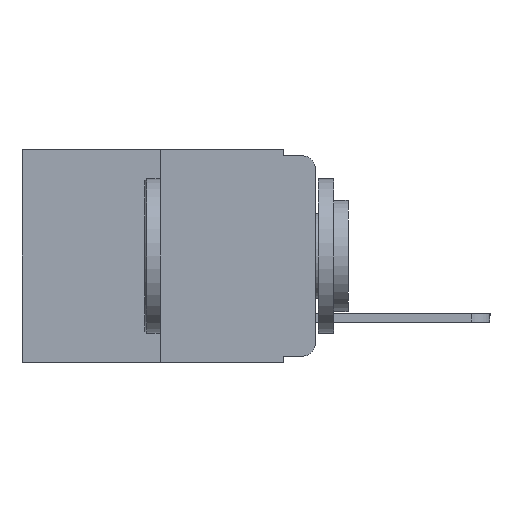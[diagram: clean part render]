
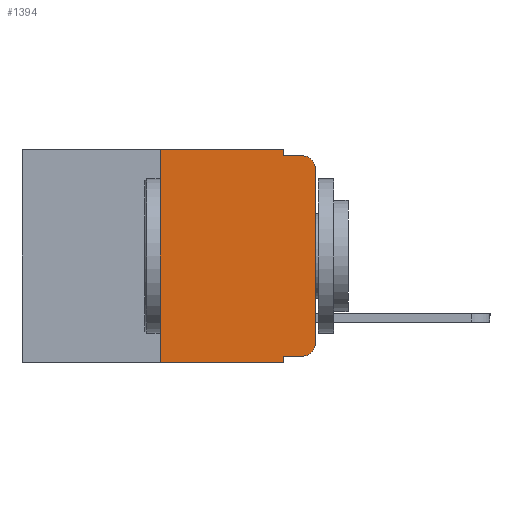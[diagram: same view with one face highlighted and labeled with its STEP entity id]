
A CAD part, left-side view. The second image highlights one B-rep face of the part: STEP entity #1394.
In plain terms, the highlighted planar face has unit normal (-1, 0, 0).
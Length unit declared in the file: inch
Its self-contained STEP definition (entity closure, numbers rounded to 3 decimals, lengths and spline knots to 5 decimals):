
#51 = CARTESIAN_POINT ( 'NONE',  ( 0., 0.051, -0.333 ) ) ;
#210 = EDGE_CURVE ( 'NONE', #1624, #1306, #15572, .T. ) ;
#361 = DIRECTION ( 'NONE',  ( 0., -1., 0. ) ) ;
#1216 = EDGE_CURVE ( 'NONE', #1306, #7808, #3694, .T. ) ;
#1306 = VERTEX_POINT ( 'NONE', #14944 ) ;
#1387 = DIRECTION ( 'NONE',  ( -1., 0., 0. ) ) ;
#1394 = ADVANCED_FACE ( 'NONE', ( #12796 ), #8373, .F. ) ;
#1551 = VERTEX_POINT ( 'NONE', #9295 ) ;
#1624 = VERTEX_POINT ( 'NONE', #13946 ) ;
#1901 = CARTESIAN_POINT ( 'NONE',  ( 0., 0., -0.03 ) ) ;
#1921 = VERTEX_POINT ( 'NONE', #14978 ) ;
#2277 = VERTEX_POINT ( 'NONE', #6408 ) ;
#2470 = CARTESIAN_POINT ( 'NONE',  ( 0., 0.25, -0.343 ) ) ;
#3202 = VERTEX_POINT ( 'NONE', #1901 ) ;
#3694 = CIRCLE ( 'NONE', #9888, 0.02 ) ;
#3838 = DIRECTION ( 'NONE',  ( 0., -1., 0. ) ) ;
#4128 = EDGE_CURVE ( 'NONE', #7808, #3202, #12061, .T. ) ;
#4379 = CARTESIAN_POINT ( 'NONE',  ( 0., 0.051, -0.343 ) ) ;
#4823 = VERTEX_POINT ( 'NONE', #4379 ) ;
#4989 = VERTEX_POINT ( 'NONE', #11772 ) ;
#5062 = LINE ( 'NONE', #13606, #20707 ) ;
#6408 = CARTESIAN_POINT ( 'NONE',  ( 0., 0.051, -0.01 ) ) ;
#6953 = DIRECTION ( 'NONE',  ( 0., -1., 0. ) ) ;
#7467 = DIRECTION ( 'NONE',  ( 0., -1., 0. ) ) ;
#7548 = EDGE_CURVE ( 'NONE', #8425, #4823, #14599, .T. ) ;
#7808 = VERTEX_POINT ( 'NONE', #11474 ) ;
#7909 = VECTOR ( 'NONE', #17127, 39.37008 ) ;
#7979 = CIRCLE ( 'NONE', #13161, 0.02 ) ;
#8373 = PLANE ( 'NONE',  #13572 ) ;
#8418 = VECTOR ( 'NONE', #6953, 39.37008 ) ;
#8425 = VERTEX_POINT ( 'NONE', #2470 ) ;
#8596 = EDGE_CURVE ( 'NONE', #2277, #1921, #5062, .T. ) ;
#8642 = CARTESIAN_POINT ( 'NONE',  ( 0., 0.473, 0. ) ) ;
#9066 = LINE ( 'NONE', #17941, #16503 ) ;
#9295 = CARTESIAN_POINT ( 'NONE',  ( 0., 0.25, 0. ) ) ;
#9774 = CARTESIAN_POINT ( 'NONE',  ( 0., 0., 0. ) ) ;
#9883 = EDGE_CURVE ( 'NONE', #1624, #4823, #9066, .T. ) ;
#9888 = AXIS2_PLACEMENT_3D ( 'NONE', #16943, #16154, #15455 ) ;
#10025 = EDGE_LOOP ( 'NONE', ( #12259, #12470, #12678, #12743, #12898, #12948, #13164, #13176, #13274, #13367 ) ) ;
#10623 = VECTOR ( 'NONE', #361, 39.37008 ) ;
#10733 = VECTOR ( 'NONE', #18582, 39.37008 ) ;
#10994 = CARTESIAN_POINT ( 'NONE',  ( 0., 0.473, -0.343 ) ) ;
#11474 = CARTESIAN_POINT ( 'NONE',  ( 0., 0., -0.313 ) ) ;
#11691 = VECTOR ( 'NONE', #3838, 39.37008 ) ;
#11772 = CARTESIAN_POINT ( 'NONE',  ( 0., 0.051, 0. ) ) ;
#11783 = CARTESIAN_POINT ( 'NONE',  ( 0., 0.02, -0.03 ) ) ;
#12061 = LINE ( 'NONE', #9774, #7909 ) ;
#12259 = ORIENTED_EDGE ( 'NONE', *, *, #4128, .T. ) ;
#12345 = VECTOR ( 'NONE', #13109, 39.37008 ) ;
#12470 = ORIENTED_EDGE ( 'NONE', *, *, #18133, .T. ) ;
#12678 = ORIENTED_EDGE ( 'NONE', *, *, #8596, .F. ) ;
#12743 = ORIENTED_EDGE ( 'NONE', *, *, #16344, .F. ) ;
#12796 = FACE_OUTER_BOUND ( 'NONE', #10025, .T. ) ;
#12810 = LINE ( 'NONE', #20193, #12345 ) ;
#12898 = ORIENTED_EDGE ( 'NONE', *, *, #19714, .F. ) ;
#12948 = ORIENTED_EDGE ( 'NONE', *, *, #17063, .F. ) ;
#13001 = LINE ( 'NONE', #8642, #8418 ) ;
#13109 = DIRECTION ( 'NONE',  ( 0., 0., -1. ) ) ;
#13132 = CARTESIAN_POINT ( 'NONE',  ( 0., 0.473, 0. ) ) ;
#13161 = AXIS2_PLACEMENT_3D ( 'NONE', #11783, #1387, #13255 ) ;
#13164 = ORIENTED_EDGE ( 'NONE', *, *, #7548, .T. ) ;
#13176 = ORIENTED_EDGE ( 'NONE', *, *, #9883, .F. ) ;
#13231 = DIRECTION ( 'NONE',  ( 0., 0., -1. ) ) ;
#13255 = DIRECTION ( 'NONE',  ( 0., 0., -1. ) ) ;
#13274 = ORIENTED_EDGE ( 'NONE', *, *, #210, .T. ) ;
#13367 = ORIENTED_EDGE ( 'NONE', *, *, #1216, .T. ) ;
#13572 = AXIS2_PLACEMENT_3D ( 'NONE', #13132, #18509, #13231 ) ;
#13606 = CARTESIAN_POINT ( 'NONE',  ( 0., 0.051, -0.01 ) ) ;
#13946 = CARTESIAN_POINT ( 'NONE',  ( 0., 0.051, -0.333 ) ) ;
#14599 = LINE ( 'NONE', #10994, #10623 ) ;
#14700 = LINE ( 'NONE', #19989, #10733 ) ;
#14944 = CARTESIAN_POINT ( 'NONE',  ( 0., 0.02, -0.333 ) ) ;
#14978 = CARTESIAN_POINT ( 'NONE',  ( 0., 0.02, -0.01 ) ) ;
#15455 = DIRECTION ( 'NONE',  ( 0., 0., -1. ) ) ;
#15572 = LINE ( 'NONE', #51, #11691 ) ;
#16154 = DIRECTION ( 'NONE',  ( -1., 0., 0. ) ) ;
#16344 = EDGE_CURVE ( 'NONE', #4989, #2277, #12810, .T. ) ;
#16503 = VECTOR ( 'NONE', #19349, 39.37008 ) ;
#16943 = CARTESIAN_POINT ( 'NONE',  ( 0., 0.02, -0.313 ) ) ;
#17063 = EDGE_CURVE ( 'NONE', #8425, #1551, #14700, .T. ) ;
#17127 = DIRECTION ( 'NONE',  ( 0., 0., 1. ) ) ;
#17941 = CARTESIAN_POINT ( 'NONE',  ( 0., 0.051, 0. ) ) ;
#18133 = EDGE_CURVE ( 'NONE', #3202, #1921, #7979, .T. ) ;
#18509 = DIRECTION ( 'NONE',  ( 1., 0., 0. ) ) ;
#18582 = DIRECTION ( 'NONE',  ( 0., 0., 1. ) ) ;
#19349 = DIRECTION ( 'NONE',  ( 0., 0., -1. ) ) ;
#19714 = EDGE_CURVE ( 'NONE', #1551, #4989, #13001, .T. ) ;
#19989 = CARTESIAN_POINT ( 'NONE',  ( 0., 0.25, 0. ) ) ;
#20193 = CARTESIAN_POINT ( 'NONE',  ( 0., 0.051, 0. ) ) ;
#20707 = VECTOR ( 'NONE', #7467, 39.37008 ) ;
